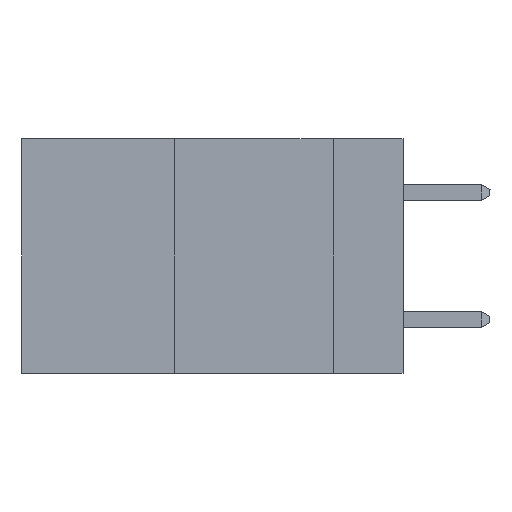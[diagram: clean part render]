
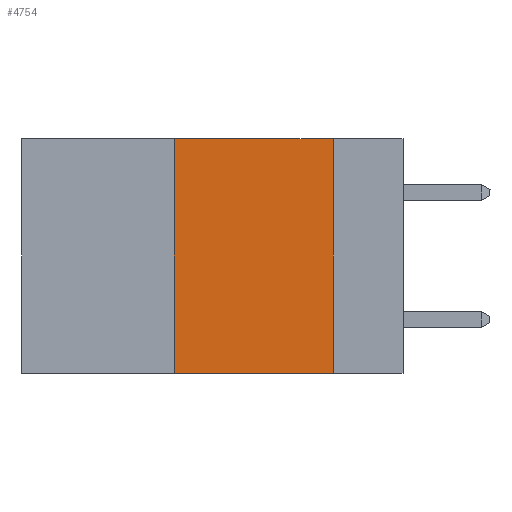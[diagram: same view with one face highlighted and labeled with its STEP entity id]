
A CAD part, left-side view. The second image highlights one B-rep face of the part: STEP entity #4754.
In plain terms, the highlighted planar face has unit normal (-1, 0, 0).
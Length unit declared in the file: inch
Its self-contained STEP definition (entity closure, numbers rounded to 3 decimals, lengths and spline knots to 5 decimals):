
#198 = VECTOR ( 'NONE', #5394, 39.37008 ) ;
#611 = CARTESIAN_POINT ( 'NONE',  ( 0., 0.11, 0. ) ) ;
#3323 = EDGE_LOOP ( 'NONE', ( #28339, #27707, #25147, #13014 ) ) ;
#4056 = DIRECTION ( 'NONE',  ( 0., -1., 0. ) ) ;
#4323 = CARTESIAN_POINT ( 'NONE',  ( 0., 0.6, 0. ) ) ;
#4348 = EDGE_CURVE ( 'NONE', #20305, #29115, #13638, .T. ) ;
#4353 = EDGE_CURVE ( 'NONE', #6244, #20305, #8858, .T. ) ;
#4754 = ADVANCED_FACE ( 'NONE', ( #8830 ), #20083, .F. ) ;
#4935 = CARTESIAN_POINT ( 'NONE',  ( 0., 0.36, 0. ) ) ;
#4944 = CARTESIAN_POINT ( 'NONE',  ( 0., 0.6, -0.37 ) ) ;
#5394 = DIRECTION ( 'NONE',  ( 0., -1., 0. ) ) ;
#6244 = VERTEX_POINT ( 'NONE', #12842 ) ;
#8830 = FACE_OUTER_BOUND ( 'NONE', #3323, .T. ) ;
#8858 = LINE ( 'NONE', #4935, #18810 ) ;
#9604 = DIRECTION ( 'NONE',  ( 0., 0., 1. ) ) ;
#10310 = DIRECTION ( 'NONE',  ( 0., 0., -1. ) ) ;
#11701 = LINE ( 'NONE', #4944, #198 ) ;
#12516 = CARTESIAN_POINT ( 'NONE',  ( 0., 0.11, -0.37 ) ) ;
#12842 = CARTESIAN_POINT ( 'NONE',  ( 0., 0.36, -0.37 ) ) ;
#13014 = ORIENTED_EDGE ( 'NONE', *, *, #19244, .T. ) ;
#13470 = DIRECTION ( 'NONE',  ( 0., 0., -1. ) ) ;
#13638 = LINE ( 'NONE', #24619, #16399 ) ;
#15571 = EDGE_CURVE ( 'NONE', #29115, #28422, #26664, .T. ) ;
#16399 = VECTOR ( 'NONE', #4056, 39.37008 ) ;
#18810 = VECTOR ( 'NONE', #9604, 39.37008 ) ;
#19244 = EDGE_CURVE ( 'NONE', #6244, #28422, #11701, .T. ) ;
#19283 = CARTESIAN_POINT ( 'NONE',  ( 0., 0.36, 0. ) ) ;
#20083 = PLANE ( 'NONE',  #21744 ) ;
#20174 = VECTOR ( 'NONE', #10310, 39.37008 ) ;
#20305 = VERTEX_POINT ( 'NONE', #19283 ) ;
#21744 = AXIS2_PLACEMENT_3D ( 'NONE', #4323, #26986, #13470 ) ;
#21877 = CARTESIAN_POINT ( 'NONE',  ( 0., 0.11, 0. ) ) ;
#24619 = CARTESIAN_POINT ( 'NONE',  ( 0., 0.6, 0. ) ) ;
#25147 = ORIENTED_EDGE ( 'NONE', *, *, #4353, .F. ) ;
#26664 = LINE ( 'NONE', #21877, #20174 ) ;
#26986 = DIRECTION ( 'NONE',  ( 1., 0., 0. ) ) ;
#27707 = ORIENTED_EDGE ( 'NONE', *, *, #4348, .F. ) ;
#28339 = ORIENTED_EDGE ( 'NONE', *, *, #15571, .F. ) ;
#28422 = VERTEX_POINT ( 'NONE', #12516 ) ;
#29115 = VERTEX_POINT ( 'NONE', #611 ) ;
